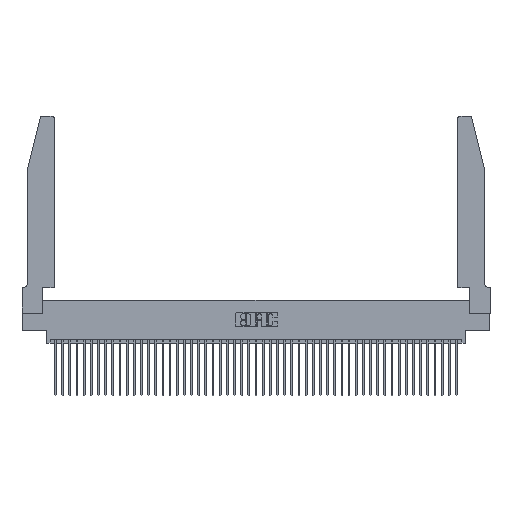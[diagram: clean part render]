
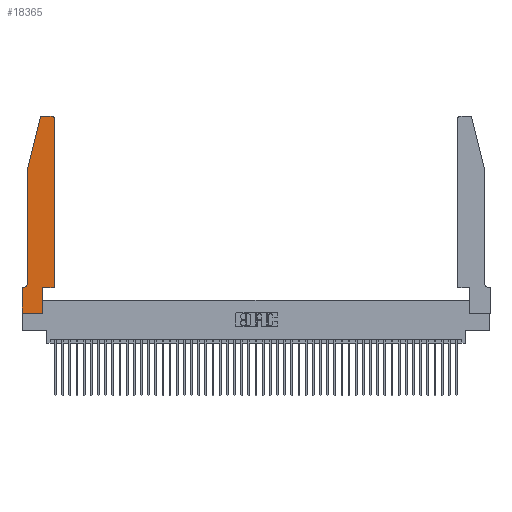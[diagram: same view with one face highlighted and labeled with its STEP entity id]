
A CAD part, top view. The second image highlights one B-rep face of the part: STEP entity #18365.
In plain terms, the highlighted planar face has unit normal (0, 0, 1).
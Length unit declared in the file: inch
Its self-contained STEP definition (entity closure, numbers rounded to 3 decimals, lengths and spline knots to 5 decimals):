
#856 = EDGE_CURVE ( 'NONE', #27925, #41306, #35547, .T. ) ;
#907 = ORIENTED_EDGE ( 'NONE', *, *, #41121, .T. ) ;
#1274 = AXIS2_PLACEMENT_3D ( 'NONE', #45186, #8738, #19698 ) ;
#1394 = CARTESIAN_POINT ( 'NONE',  ( 0.2865, 0.35, 0.37 ) ) ;
#1686 = EDGE_CURVE ( 'NONE', #13643, #47293, #7892, .T. ) ;
#1692 = VECTOR ( 'NONE', #34251, 39.37008 ) ;
#1743 = CARTESIAN_POINT ( 'NONE',  ( 0., 0., 0.37 ) ) ;
#1765 = DIRECTION ( 'NONE',  ( 0., 0., 1. ) ) ;
#1946 = ORIENTED_EDGE ( 'NONE', *, *, #856, .T. ) ;
#1979 = VECTOR ( 'NONE', #36787, 39.37008 ) ;
#2665 = FACE_OUTER_BOUND ( 'NONE', #33197, .T. ) ;
#3329 = VERTEX_POINT ( 'NONE', #19487 ) ;
#3465 = ORIENTED_EDGE ( 'NONE', *, *, #31556, .T. ) ;
#3872 = VECTOR ( 'NONE', #31854, 39.37008 ) ;
#4336 = ORIENTED_EDGE ( 'NONE', *, *, #42382, .T. ) ;
#4481 = VECTOR ( 'NONE', #35655, 39.37008 ) ;
#4897 = DIRECTION ( 'NONE',  ( 1., 0., 0. ) ) ;
#5272 = ORIENTED_EDGE ( 'NONE', *, *, #38947, .T. ) ;
#5650 = CARTESIAN_POINT ( 'NONE',  ( 0., 0., 0.37 ) ) ;
#7401 = CARTESIAN_POINT ( 'NONE',  ( 0.0755, 0.35, 0.37 ) ) ;
#7892 = LINE ( 'NONE', #45539, #3872 ) ;
#8585 = CARTESIAN_POINT ( 'NONE',  ( 0.0755, 2., 0.37 ) ) ;
#8738 = DIRECTION ( 'NONE',  ( 0., 0., 1. ) ) ;
#9239 = DIRECTION ( 'NONE',  ( -1., 0., 0. ) ) ;
#9375 = ORIENTED_EDGE ( 'NONE', *, *, #14091, .T. ) ;
#10933 = VECTOR ( 'NONE', #20903, 39.37008 ) ;
#10957 = LINE ( 'NONE', #34397, #14978 ) ;
#11211 = CARTESIAN_POINT ( 'NONE',  ( 0.25487, 2.72718, 0.37 ) ) ;
#12831 = CARTESIAN_POINT ( 'NONE',  ( 0.0755, 0.42, 0.37 ) ) ;
#13243 = CARTESIAN_POINT ( 'NONE',  ( 0.4505, 2.72, 0.37 ) ) ;
#13637 = DIRECTION ( 'NONE',  ( -1., 0., 0. ) ) ;
#13643 = VERTEX_POINT ( 'NONE', #1743 ) ;
#14091 = EDGE_CURVE ( 'NONE', #3329, #43236, #33499, .T. ) ;
#14978 = VECTOR ( 'NONE', #9239, 39.37008 ) ;
#15765 = CARTESIAN_POINT ( 'NONE',  ( 0.0055, 0.35, 0.37 ) ) ;
#16833 = VERTEX_POINT ( 'NONE', #39821 ) ;
#17815 = VERTEX_POINT ( 'NONE', #23865 ) ;
#18001 = ORIENTED_EDGE ( 'NONE', *, *, #45036, .T. ) ;
#18300 = DIRECTION ( 'NONE',  ( -1., 0., 0. ) ) ;
#18365 = ADVANCED_FACE ( 'NONE', ( #2665 ), #44402, .T. ) ;
#19487 = CARTESIAN_POINT ( 'NONE',  ( 0.284, 2.75, 0.37 ) ) ;
#19698 = DIRECTION ( 'NONE',  ( 1., 0., 0. ) ) ;
#19843 = ORIENTED_EDGE ( 'NONE', *, *, #30907, .T. ) ;
#19964 = EDGE_CURVE ( 'NONE', #25648, #17815, #36503, .T. ) ;
#20337 = EDGE_CURVE ( 'NONE', #41306, #24632, #42827, .T. ) ;
#20508 = AXIS2_PLACEMENT_3D ( 'NONE', #41980, #1765, #34541 ) ;
#20535 = AXIS2_PLACEMENT_3D ( 'NONE', #26970, #22784, #4897 ) ;
#20657 = DIRECTION ( 'NONE',  ( 0., -1., 0. ) ) ;
#20700 = CARTESIAN_POINT ( 'NONE',  ( 0.2865, 0.35, 0.37 ) ) ;
#20903 = DIRECTION ( 'NONE',  ( -0.239, -0.971, 0. ) ) ;
#21227 = LINE ( 'NONE', #8585, #1692 ) ;
#22498 = CIRCLE ( 'NONE', #41118, 0.07 ) ;
#22525 = CARTESIAN_POINT ( 'NONE',  ( 0.4505, 0.35, 0.37 ) ) ;
#22784 = DIRECTION ( 'NONE',  ( 0., 0., 1. ) ) ;
#23518 = EDGE_CURVE ( 'NONE', #46225, #3329, #10957, .T. ) ;
#23865 = CARTESIAN_POINT ( 'NONE',  ( 0., 0.35, 0.37 ) ) ;
#24632 = VERTEX_POINT ( 'NONE', #13243 ) ;
#25648 = VERTEX_POINT ( 'NONE', #15765 ) ;
#26663 = VERTEX_POINT ( 'NONE', #12831 ) ;
#26960 = CARTESIAN_POINT ( 'NONE',  ( 0.2865, 0., 0.37 ) ) ;
#26970 = CARTESIAN_POINT ( 'NONE',  ( 0., 0.35, 0.37 ) ) ;
#27818 = CARTESIAN_POINT ( 'NONE',  ( 0.4505, 0.35, 0.37 ) ) ;
#27925 = VERTEX_POINT ( 'NONE', #1394 ) ;
#29241 = VECTOR ( 'NONE', #35365, 39.37008 ) ;
#29347 = ORIENTED_EDGE ( 'NONE', *, *, #20337, .T. ) ;
#30907 = EDGE_CURVE ( 'NONE', #24632, #46225, #41831, .T. ) ;
#31503 = ORIENTED_EDGE ( 'NONE', *, *, #1686, .T. ) ;
#31556 = EDGE_CURVE ( 'NONE', #17815, #13643, #39250, .T. ) ;
#31682 = VECTOR ( 'NONE', #20657, 39.37008 ) ;
#31854 = DIRECTION ( 'NONE',  ( 1., 0., 0. ) ) ;
#33197 = EDGE_LOOP ( 'NONE', ( #36436, #9375, #18001, #907, #5272, #47236, #3465, #31503, #4336, #1946, #29347, #19843 ) ) ;
#33499 = CIRCLE ( 'NONE', #1274, 0.03 ) ;
#34251 = DIRECTION ( 'NONE',  ( 0., -1., 0. ) ) ;
#34397 = CARTESIAN_POINT ( 'NONE',  ( 0.2605, 2.75, 0.37 ) ) ;
#34541 = DIRECTION ( 'NONE',  ( 1., 0., 0. ) ) ;
#34977 = CARTESIAN_POINT ( 'NONE',  ( 0.4505, 0.35, 0.37 ) ) ;
#35365 = DIRECTION ( 'NONE',  ( 1., 0., 0. ) ) ;
#35547 = LINE ( 'NONE', #27818, #29241 ) ;
#35655 = DIRECTION ( 'NONE',  ( 0., 1., 0. ) ) ;
#36436 = ORIENTED_EDGE ( 'NONE', *, *, #23518, .T. ) ;
#36503 = LINE ( 'NONE', #7401, #47512 ) ;
#36787 = DIRECTION ( 'NONE',  ( 0., 1., 0. ) ) ;
#38174 = CARTESIAN_POINT ( 'NONE',  ( 0.4205, 2.75, 0.37 ) ) ;
#38947 = EDGE_CURVE ( 'NONE', #26663, #25648, #22498, .T. ) ;
#39250 = LINE ( 'NONE', #5650, #31682 ) ;
#39704 = LINE ( 'NONE', #43603, #10933 ) ;
#39821 = CARTESIAN_POINT ( 'NONE',  ( 0.0755, 2., 0.37 ) ) ;
#39966 = CARTESIAN_POINT ( 'NONE',  ( 0.0055, 0.42, 0.37 ) ) ;
#41118 = AXIS2_PLACEMENT_3D ( 'NONE', #39966, #43169, #13637 ) ;
#41121 = EDGE_CURVE ( 'NONE', #16833, #26663, #21227, .T. ) ;
#41306 = VERTEX_POINT ( 'NONE', #22525 ) ;
#41831 = CIRCLE ( 'NONE', #20508, 0.03 ) ;
#41980 = CARTESIAN_POINT ( 'NONE',  ( 0.4205, 2.72, 0.37 ) ) ;
#42382 = EDGE_CURVE ( 'NONE', #47293, #27925, #44713, .T. ) ;
#42827 = LINE ( 'NONE', #34977, #1979 ) ;
#43169 = DIRECTION ( 'NONE',  ( 0., 0., -1. ) ) ;
#43236 = VERTEX_POINT ( 'NONE', #11211 ) ;
#43603 = CARTESIAN_POINT ( 'NONE',  ( 0.0755, 2., 0.37 ) ) ;
#44402 = PLANE ( 'NONE',  #20535 ) ;
#44713 = LINE ( 'NONE', #20700, #4481 ) ;
#45036 = EDGE_CURVE ( 'NONE', #43236, #16833, #39704, .T. ) ;
#45186 = CARTESIAN_POINT ( 'NONE',  ( 0.284, 2.72, 0.37 ) ) ;
#45539 = CARTESIAN_POINT ( 'NONE',  ( 0., 0., 0.37 ) ) ;
#46225 = VERTEX_POINT ( 'NONE', #38174 ) ;
#47236 = ORIENTED_EDGE ( 'NONE', *, *, #19964, .T. ) ;
#47293 = VERTEX_POINT ( 'NONE', #26960 ) ;
#47512 = VECTOR ( 'NONE', #18300, 39.37008 ) ;
